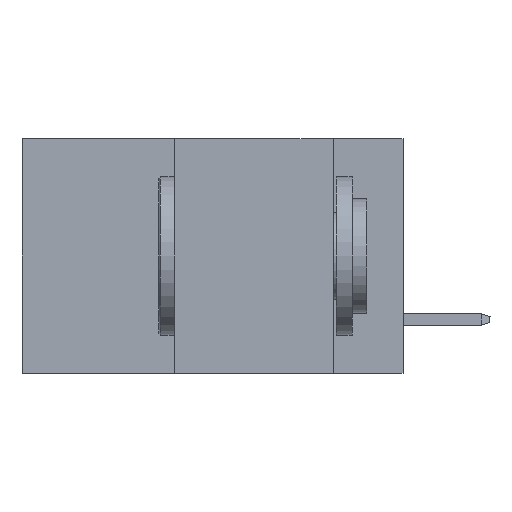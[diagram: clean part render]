
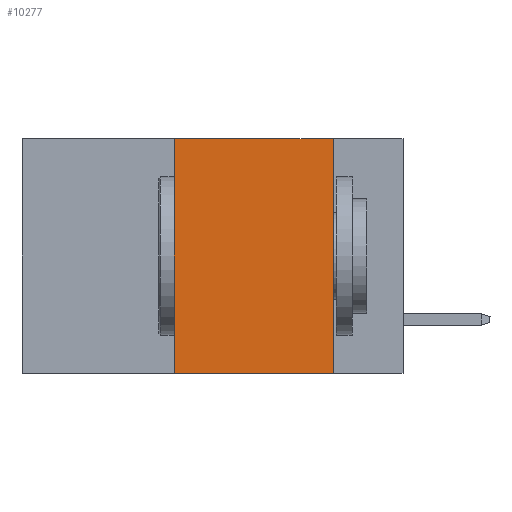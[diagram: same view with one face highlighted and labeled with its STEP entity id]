
A CAD part, left-side view. The second image highlights one B-rep face of the part: STEP entity #10277.
In plain terms, the highlighted planar face has unit normal (-1, 0, 0).
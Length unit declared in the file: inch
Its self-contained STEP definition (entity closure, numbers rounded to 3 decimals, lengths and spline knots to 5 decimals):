
#693 = EDGE_CURVE ( 'NONE', #9750, #11601, #5804, .T. ) ;
#999 = DIRECTION ( 'NONE',  ( 1., 0., 0. ) ) ;
#1601 = ORIENTED_EDGE ( 'NONE', *, *, #9551, .F. ) ;
#2164 = ORIENTED_EDGE ( 'NONE', *, *, #8464, .T. ) ;
#2366 = VERTEX_POINT ( 'NONE', #10007 ) ;
#2678 = CARTESIAN_POINT ( 'NONE',  ( 0., 0.36, 0. ) ) ;
#2929 = VECTOR ( 'NONE', #3813, 39.37008 ) ;
#3813 = DIRECTION ( 'NONE',  ( 0., -1., 0. ) ) ;
#3887 = DIRECTION ( 'NONE',  ( 0., 0., 1. ) ) ;
#4088 = VERTEX_POINT ( 'NONE', #9954 ) ;
#4226 = FACE_OUTER_BOUND ( 'NONE', #10583, .T. ) ;
#4449 = CARTESIAN_POINT ( 'NONE',  ( 0., 0.6, -0.37 ) ) ;
#5442 = CARTESIAN_POINT ( 'NONE',  ( 0., 0.11, 0. ) ) ;
#5622 = DIRECTION ( 'NONE',  ( 0., 0., -1. ) ) ;
#5804 = LINE ( 'NONE', #9487, #2929 ) ;
#7858 = LINE ( 'NONE', #10525, #10112 ) ;
#8464 = EDGE_CURVE ( 'NONE', #2366, #4088, #11261, .T. ) ;
#8707 = LINE ( 'NONE', #2678, #9365 ) ;
#8976 = VECTOR ( 'NONE', #11328, 39.37008 ) ;
#8985 = PLANE ( 'NONE',  #11128 ) ;
#9170 = ORIENTED_EDGE ( 'NONE', *, *, #693, .F. ) ;
#9365 = VECTOR ( 'NONE', #3887, 39.37008 ) ;
#9487 = CARTESIAN_POINT ( 'NONE',  ( 0., 0.6, 0. ) ) ;
#9551 = EDGE_CURVE ( 'NONE', #11601, #4088, #7858, .T. ) ;
#9750 = VERTEX_POINT ( 'NONE', #10671 ) ;
#9815 = CARTESIAN_POINT ( 'NONE',  ( 0., 0.6, 0. ) ) ;
#9954 = CARTESIAN_POINT ( 'NONE',  ( 0., 0.11, -0.37 ) ) ;
#10007 = CARTESIAN_POINT ( 'NONE',  ( 0., 0.36, -0.37 ) ) ;
#10112 = VECTOR ( 'NONE', #5622, 39.37008 ) ;
#10277 = ADVANCED_FACE ( 'NONE', ( #4226 ), #8985, .F. ) ;
#10525 = CARTESIAN_POINT ( 'NONE',  ( 0., 0.11, 0. ) ) ;
#10583 = EDGE_LOOP ( 'NONE', ( #1601, #9170, #12113, #2164 ) ) ;
#10671 = CARTESIAN_POINT ( 'NONE',  ( 0., 0.36, 0. ) ) ;
#11128 = AXIS2_PLACEMENT_3D ( 'NONE', #9815, #999, #12018 ) ;
#11261 = LINE ( 'NONE', #4449, #8976 ) ;
#11328 = DIRECTION ( 'NONE',  ( 0., -1., 0. ) ) ;
#11601 = VERTEX_POINT ( 'NONE', #5442 ) ;
#11794 = EDGE_CURVE ( 'NONE', #2366, #9750, #8707, .T. ) ;
#12018 = DIRECTION ( 'NONE',  ( 0., 0., -1. ) ) ;
#12113 = ORIENTED_EDGE ( 'NONE', *, *, #11794, .F. ) ;
